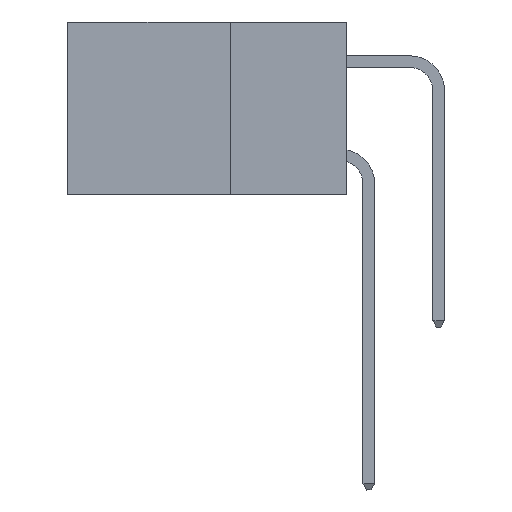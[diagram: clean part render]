
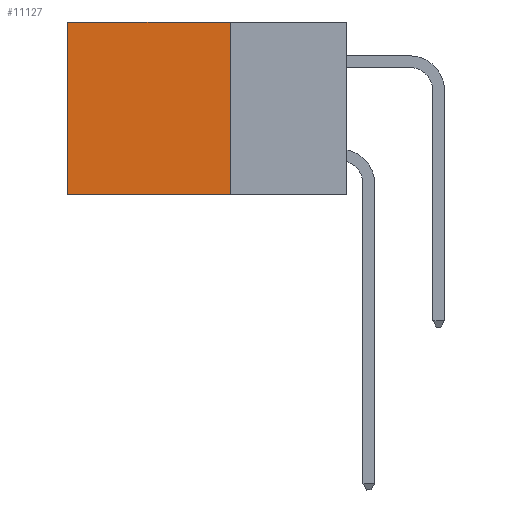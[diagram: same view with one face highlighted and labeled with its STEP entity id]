
A CAD part, left-side view. The second image highlights one B-rep face of the part: STEP entity #11127.
In plain terms, the highlighted planar face has unit normal (-1, 0, 0).
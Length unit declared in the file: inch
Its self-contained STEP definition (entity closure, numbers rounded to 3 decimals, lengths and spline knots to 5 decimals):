
#556 = CARTESIAN_POINT ( 'NONE',  ( 0.2875, 0.25, -0.37 ) ) ;
#753 = ORIENTED_EDGE ( 'NONE', *, *, #16667, .T. ) ;
#1011 = VECTOR ( 'NONE', #20891, 39.37008 ) ;
#1100 = CARTESIAN_POINT ( 'NONE',  ( 0.2875, 0.6, 0. ) ) ;
#1188 = LINE ( 'NONE', #556, #7190 ) ;
#1338 = DIRECTION ( 'NONE',  ( 0., 0., -1. ) ) ;
#3436 = ORIENTED_EDGE ( 'NONE', *, *, #12827, .F. ) ;
#3490 = PLANE ( 'NONE',  #19586 ) ;
#4791 = VERTEX_POINT ( 'NONE', #9622 ) ;
#5119 = VERTEX_POINT ( 'NONE', #8896 ) ;
#5211 = ORIENTED_EDGE ( 'NONE', *, *, #14682, .F. ) ;
#6316 = EDGE_LOOP ( 'NONE', ( #18765, #5211, #3436, #753 ) ) ;
#6379 = VERTEX_POINT ( 'NONE', #11480 ) ;
#6601 = CARTESIAN_POINT ( 'NONE',  ( 0.2875, 0.25, 0. ) ) ;
#7190 = VECTOR ( 'NONE', #9697, 39.37008 ) ;
#8896 = CARTESIAN_POINT ( 'NONE',  ( 0.2875, 0.6, -0.37 ) ) ;
#9622 = CARTESIAN_POINT ( 'NONE',  ( 0.2875, 0.25, 0. ) ) ;
#9697 = DIRECTION ( 'NONE',  ( 0., 1., 0. ) ) ;
#10865 = CARTESIAN_POINT ( 'NONE',  ( 0.2875, 0.25, 0. ) ) ;
#11127 = ADVANCED_FACE ( 'NONE', ( #12619 ), #3490, .F. ) ;
#11243 = LINE ( 'NONE', #17188, #1011 ) ;
#11480 = CARTESIAN_POINT ( 'NONE',  ( 0.2875, 0.6, 0. ) ) ;
#11935 = DIRECTION ( 'NONE',  ( 0., 1., 0. ) ) ;
#12619 = FACE_OUTER_BOUND ( 'NONE', #6316, .T. ) ;
#12753 = LINE ( 'NONE', #6601, #14725 ) ;
#12827 = EDGE_CURVE ( 'NONE', #4791, #16232, #11243, .T. ) ;
#13796 = LINE ( 'NONE', #1100, #14063 ) ;
#14063 = VECTOR ( 'NONE', #1338, 39.37008 ) ;
#14682 = EDGE_CURVE ( 'NONE', #16232, #5119, #1188, .T. ) ;
#14725 = VECTOR ( 'NONE', #11935, 39.37008 ) ;
#16232 = VERTEX_POINT ( 'NONE', #21341 ) ;
#16287 = DIRECTION ( 'NONE',  ( 1., 0., 0. ) ) ;
#16667 = EDGE_CURVE ( 'NONE', #4791, #6379, #12753, .T. ) ;
#17188 = CARTESIAN_POINT ( 'NONE',  ( 0.2875, 0.25, 0. ) ) ;
#18257 = DIRECTION ( 'NONE',  ( 0., 0., -1. ) ) ;
#18765 = ORIENTED_EDGE ( 'NONE', *, *, #22568, .T. ) ;
#19586 = AXIS2_PLACEMENT_3D ( 'NONE', #10865, #16287, #18257 ) ;
#20891 = DIRECTION ( 'NONE',  ( 0., 0., -1. ) ) ;
#21341 = CARTESIAN_POINT ( 'NONE',  ( 0.2875, 0.25, -0.37 ) ) ;
#22568 = EDGE_CURVE ( 'NONE', #6379, #5119, #13796, .T. ) ;
